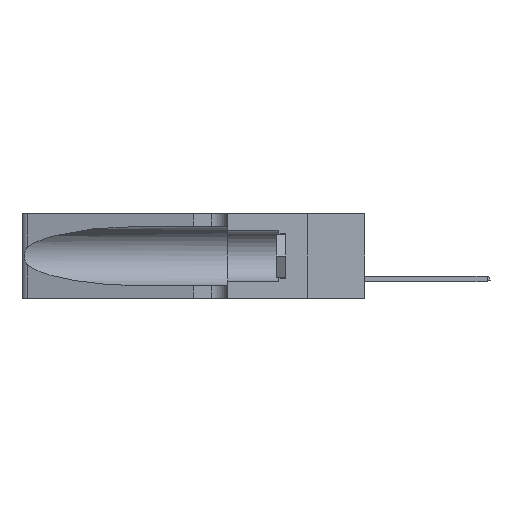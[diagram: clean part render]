
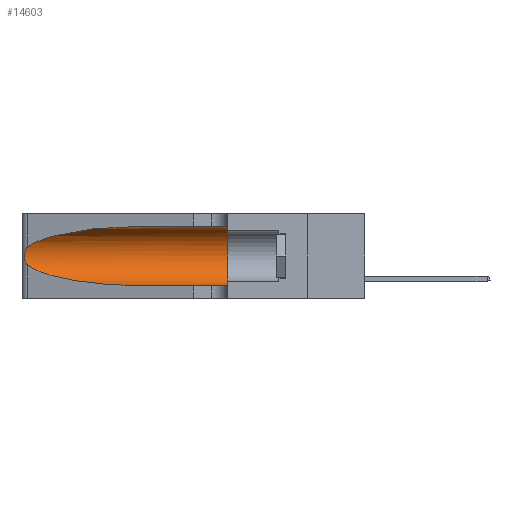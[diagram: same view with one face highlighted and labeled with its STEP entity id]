
A CAD part, left-side view. The second image highlights one B-rep face of the part: STEP entity #14603.
In plain terms, the highlighted cylindrical face has radius 3.308 mm (diameter 6.617 mm), a partial arc.
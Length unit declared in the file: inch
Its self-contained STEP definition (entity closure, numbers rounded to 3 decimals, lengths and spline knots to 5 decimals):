
#103 = VERTEX_POINT ( 'NONE', #5841 ) ;
#197 = CIRCLE ( 'NONE', #21352, 0.13025 ) ;
#214 = CARTESIAN_POINT ( 'NONE',  ( 0.18966, 0.96281, 0.05475 ) ) ;
#300 = DIRECTION ( 'NONE',  ( 0., -1., 0. ) ) ;
#466 = CARTESIAN_POINT ( 'NONE',  ( 0.1305, 1.61858, 0.185 ) ) ;
#1268 = DIRECTION ( 'NONE',  ( 0., 1., 0. ) ) ;
#1622 = VECTOR ( 'NONE', #21511, 39.37008 ) ;
#1996 = CARTESIAN_POINT ( 'NONE',  ( 0.25487, 1.22718, 0.14631 ) ) ;
#2114 = EDGE_CURVE ( 'NONE', #20142, #17226, #16264, .T. ) ;
#2161 = DIRECTION ( 'NONE',  ( 0., 0., -1. ) ) ;
#2233 = CARTESIAN_POINT ( 'NONE',  ( 0.2373, 1.15595, 0.08982 ) ) ;
#2431 = CARTESIAN_POINT ( 'NONE',  ( 0.2373, 1.15595, 0.28018 ) ) ;
#4941 = VERTEX_POINT ( 'NONE', #15770 ) ;
#5267 = AXIS2_PLACEMENT_3D ( 'NONE', #466, #300, #2161 ) ;
#5754 = LINE ( 'NONE', #22459, #18707 ) ;
#5763 = EDGE_LOOP ( 'NONE', ( #6035, #22727, #17870, #14193, #9693, #15859 ) ) ;
#5824 = CARTESIAN_POINT ( 'NONE',  ( 0.25854, 1.2359, 0.20912 ) ) ;
#5841 = CARTESIAN_POINT ( 'NONE',  ( 0.1305, 0.72297, 0.31525 ) ) ;
#5903 = CARTESIAN_POINT ( 'NONE',  ( 0.25639, 1.23184, 0.21858 ) ) ;
#5931 =( BOUNDED_CURVE ( )  B_SPLINE_CURVE ( 3, ( #9970, #22765, #2431, #11730 ),
 .UNSPECIFIED., .F., .F. ) 
 B_SPLINE_CURVE_WITH_KNOTS ( ( 4, 4 ),
 ( 1.5708, 2.84003 ),
 .UNSPECIFIED. ) 
 CURVE ( )  GEOMETRIC_REPRESENTATION_ITEM ( )  RATIONAL_B_SPLINE_CURVE ( ( 1., 0.87, 0.87, 1. ) ) 
 REPRESENTATION_ITEM ( '' )  );
#6035 = ORIENTED_EDGE ( 'NONE', *, *, #7314, .T. ) ;
#6116 = EDGE_CURVE ( 'NONE', #103, #12510, #5754, .T. ) ;
#6843 = CARTESIAN_POINT ( 'NONE',  ( 0.1305, 1.61858, 0.05475 ) ) ;
#7314 = EDGE_CURVE ( 'NONE', #103, #4941, #5931, .T. ) ;
#7339 = CYLINDRICAL_SURFACE ( 'NONE', #5267, 0.13025 ) ;
#7347 = CARTESIAN_POINT ( 'NONE',  ( 0.26075, 1.23896, 0.19203 ) ) ;
#7420 = CARTESIAN_POINT ( 'NONE',  ( 0.25639, 1.23186, 0.15144 ) ) ;
#7499 = CARTESIAN_POINT ( 'NONE',  ( 0.25555, 1.22994, 0.2215 ) ) ;
#9081 = CARTESIAN_POINT ( 'NONE',  ( 0.26018, 1.23835, 0.19895 ) ) ;
#9235 = CARTESIAN_POINT ( 'NONE',  ( 0.25789, 1.23486, 0.15765 ) ) ;
#9516 = CARTESIAN_POINT ( 'NONE',  ( 0.25487, 1.22718, 0.14631 ) ) ;
#9693 = ORIENTED_EDGE ( 'NONE', *, *, #11102, .F. ) ;
#9970 = CARTESIAN_POINT ( 'NONE',  ( 0.1305, 0.72297, 0.31525 ) ) ;
#11102 = EDGE_CURVE ( 'NONE', #12510, #18045, #197, .T. ) ;
#11730 = CARTESIAN_POINT ( 'NONE',  ( 0.25487, 1.22718, 0.22369 ) ) ;
#12018 = LINE ( 'NONE', #6843, #1622 ) ;
#12510 = VERTEX_POINT ( 'NONE', #21657 ) ;
#12832 = CARTESIAN_POINT ( 'NONE',  ( 0.26017, 1.23833, 0.17102 ) ) ;
#13113 = CARTESIAN_POINT ( 'NONE',  ( 0.1305, 0.72297, 0.05475 ) ) ;
#13500 = EDGE_CURVE ( 'NONE', #17226, #18045, #12018, .T. ) ;
#13921 = EDGE_CURVE ( 'NONE', #4941, #20142, #15065, .T. ) ;
#14193 = ORIENTED_EDGE ( 'NONE', *, *, #13500, .T. ) ;
#14603 = ADVANCED_FACE ( 'NONE', ( #22637 ), #7339, .F. ) ;
#14765 = CARTESIAN_POINT ( 'NONE',  ( 0.26075, 1.23896, 0.178 ) ) ;
#15065 = B_SPLINE_CURVE_WITH_KNOTS ( 'NONE', 3,
 ( #16714, #7499, #5903, #20437, #5824, #9081, #7347, #14765, #12832, #20270, #9235, #7420, #16621, #22201 ),
 .UNSPECIFIED., .F., .F.,
 ( 4, 2, 2, 2, 2, 2, 4 ),
 ( 0., 0.00027, 0.00053, 0.00107, 0.0016, 0.00187, 0.00214 ),
 .UNSPECIFIED. ) ;
#15770 = CARTESIAN_POINT ( 'NONE',  ( 0.25487, 1.22718, 0.22369 ) ) ;
#15859 = ORIENTED_EDGE ( 'NONE', *, *, #6116, .F. ) ;
#16264 =( BOUNDED_CURVE ( )  B_SPLINE_CURVE ( 3, ( #9516, #2233, #214, #13113 ),
 .UNSPECIFIED., .F., .F. ) 
 B_SPLINE_CURVE_WITH_KNOTS ( ( 4, 4 ),
 ( 3.44316, 4.71239 ),
 .UNSPECIFIED. ) 
 CURVE ( )  GEOMETRIC_REPRESENTATION_ITEM ( )  RATIONAL_B_SPLINE_CURVE ( ( 1., 0.87, 0.87, 1. ) ) 
 REPRESENTATION_ITEM ( '' )  );
#16621 = CARTESIAN_POINT ( 'NONE',  ( 0.25555, 1.22993, 0.14849 ) ) ;
#16714 = CARTESIAN_POINT ( 'NONE',  ( 0.25487, 1.22718, 0.22369 ) ) ;
#17226 = VERTEX_POINT ( 'NONE', #17455 ) ;
#17455 = CARTESIAN_POINT ( 'NONE',  ( 0.1305, 0.72297, 0.05475 ) ) ;
#17870 = ORIENTED_EDGE ( 'NONE', *, *, #2114, .T. ) ;
#18045 = VERTEX_POINT ( 'NONE', #22043 ) ;
#18707 = VECTOR ( 'NONE', #22617, 39.37008 ) ;
#19658 = CARTESIAN_POINT ( 'NONE',  ( 0.1305, 0.35, 0.185 ) ) ;
#20142 = VERTEX_POINT ( 'NONE', #1996 ) ;
#20270 = CARTESIAN_POINT ( 'NONE',  ( 0.25856, 1.23593, 0.16098 ) ) ;
#20437 = CARTESIAN_POINT ( 'NONE',  ( 0.25787, 1.23484, 0.2124 ) ) ;
#21352 = AXIS2_PLACEMENT_3D ( 'NONE', #19658, #1268, #23520 ) ;
#21511 = DIRECTION ( 'NONE',  ( 0., -1., 0. ) ) ;
#21657 = CARTESIAN_POINT ( 'NONE',  ( 0.1305, 0.35, 0.31525 ) ) ;
#22043 = CARTESIAN_POINT ( 'NONE',  ( 0.1305, 0.35, 0.05475 ) ) ;
#22201 = CARTESIAN_POINT ( 'NONE',  ( 0.25487, 1.22718, 0.14631 ) ) ;
#22459 = CARTESIAN_POINT ( 'NONE',  ( 0.1305, 1.61858, 0.31525 ) ) ;
#22617 = DIRECTION ( 'NONE',  ( 0., -1., 0. ) ) ;
#22637 = FACE_OUTER_BOUND ( 'NONE', #5763, .T. ) ;
#22727 = ORIENTED_EDGE ( 'NONE', *, *, #13921, .T. ) ;
#22765 = CARTESIAN_POINT ( 'NONE',  ( 0.18966, 0.96281, 0.31525 ) ) ;
#23520 = DIRECTION ( 'NONE',  ( 0., 0., 1. ) ) ;
